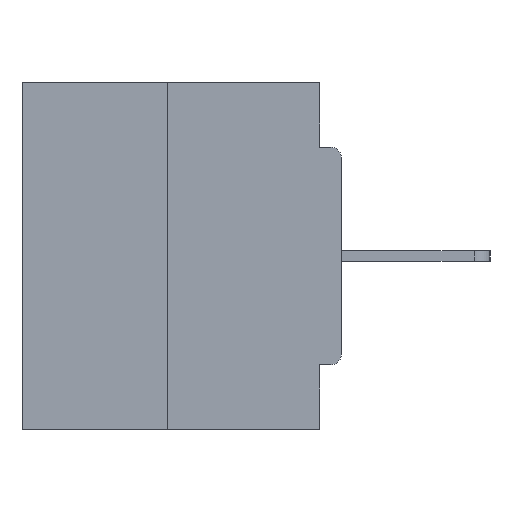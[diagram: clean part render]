
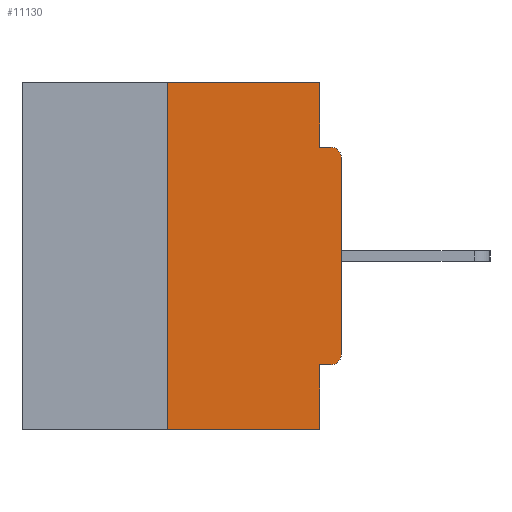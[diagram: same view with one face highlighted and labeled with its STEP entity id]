
A CAD part, left-side view. The second image highlights one B-rep face of the part: STEP entity #11130.
In plain terms, the highlighted planar face has unit normal (-1, 0, 0).
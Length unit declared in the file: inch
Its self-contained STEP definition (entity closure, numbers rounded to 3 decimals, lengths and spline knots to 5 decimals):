
#253 = CARTESIAN_POINT ( 'NONE',  ( 0., 0., 0. ) ) ;
#277 = ORIENTED_EDGE ( 'NONE', *, *, #20752, .F. ) ;
#402 = DIRECTION ( 'NONE',  ( 0., -1., 0. ) ) ;
#675 = DIRECTION ( 'NONE',  ( 0., 0., 1. ) ) ;
#771 = LINE ( 'NONE', #26077, #10764 ) ;
#1321 = VECTOR ( 'NONE', #22641, 39.37008 ) ;
#2337 = VERTEX_POINT ( 'NONE', #20572 ) ;
#3588 = CIRCLE ( 'NONE', #19612, 0.015 ) ;
#3824 = FACE_OUTER_BOUND ( 'NONE', #23256, .T. ) ;
#4654 = LINE ( 'NONE', #253, #6382 ) ;
#5637 = DIRECTION ( 'NONE',  ( 0., -1., 0. ) ) ;
#6382 = VECTOR ( 'NONE', #675, 39.37008 ) ;
#6690 = LINE ( 'NONE', #28647, #6852 ) ;
#6852 = VECTOR ( 'NONE', #22323, 39.37008 ) ;
#6928 = VERTEX_POINT ( 'NONE', #12675 ) ;
#7060 = VERTEX_POINT ( 'NONE', #24286 ) ;
#7153 = VERTEX_POINT ( 'NONE', #20764 ) ;
#8104 = ORIENTED_EDGE ( 'NONE', *, *, #13348, .F. ) ;
#8130 = DIRECTION ( 'NONE',  ( 0., 1., 0. ) ) ;
#8298 = VERTEX_POINT ( 'NONE', #16218 ) ;
#8921 = VECTOR ( 'NONE', #8130, 39.37008 ) ;
#9485 = EDGE_CURVE ( 'NONE', #28665, #2337, #20408, .T. ) ;
#10111 = DIRECTION ( 'NONE',  ( 0., 0., -1. ) ) ;
#10588 = DIRECTION ( 'NONE',  ( 0., 0., -1. ) ) ;
#10665 = CARTESIAN_POINT ( 'NONE',  ( 0., 0.015, -0.1085 ) ) ;
#10764 = VECTOR ( 'NONE', #23719, 39.37008 ) ;
#10815 = DIRECTION ( 'NONE',  ( -1., 0., 0. ) ) ;
#11130 = ADVANCED_FACE ( 'NONE', ( #3824 ), #12814, .F. ) ;
#11591 = LINE ( 'NONE', #20735, #1321 ) ;
#11714 = EDGE_CURVE ( 'NONE', #2337, #20192, #4654, .T. ) ;
#12382 = CARTESIAN_POINT ( 'NONE',  ( 0., 0.031, -0.4065 ) ) ;
#12442 = CARTESIAN_POINT ( 'NONE',  ( 0., 0.25, 0. ) ) ;
#12469 = CARTESIAN_POINT ( 'NONE',  ( 0., 0.031, -0.5 ) ) ;
#12675 = CARTESIAN_POINT ( 'NONE',  ( 0., 0.015, -0.0935 ) ) ;
#12814 = PLANE ( 'NONE',  #23311 ) ;
#12928 = ORIENTED_EDGE ( 'NONE', *, *, #11714, .T. ) ;
#13061 = EDGE_CURVE ( 'NONE', #8298, #7153, #21163, .T. ) ;
#13192 = DIRECTION ( 'NONE',  ( 0., 0., -1. ) ) ;
#13348 = EDGE_CURVE ( 'NONE', #20266, #7060, #6690, .T. ) ;
#13528 = ORIENTED_EDGE ( 'NONE', *, *, #24818, .F. ) ;
#14208 = ORIENTED_EDGE ( 'NONE', *, *, #13061, .T. ) ;
#14288 = AXIS2_PLACEMENT_3D ( 'NONE', #15085, #24336, #15395 ) ;
#14885 = CARTESIAN_POINT ( 'NONE',  ( 0., 0.46, 0. ) ) ;
#15014 = ORIENTED_EDGE ( 'NONE', *, *, #9485, .T. ) ;
#15085 = CARTESIAN_POINT ( 'NONE',  ( 0., 0.015, -0.3915 ) ) ;
#15395 = DIRECTION ( 'NONE',  ( 0., 0., -1. ) ) ;
#16218 = CARTESIAN_POINT ( 'NONE',  ( 0., 0.25, -0.5 ) ) ;
#16413 = CARTESIAN_POINT ( 'NONE',  ( 0., 0., -0.0935 ) ) ;
#18247 = CARTESIAN_POINT ( 'NONE',  ( 0., 0.46, -0.5 ) ) ;
#18319 = ORIENTED_EDGE ( 'NONE', *, *, #21670, .T. ) ;
#18381 = ORIENTED_EDGE ( 'NONE', *, *, #23871, .F. ) ;
#18472 = LINE ( 'NONE', #16413, #22472 ) ;
#19612 = AXIS2_PLACEMENT_3D ( 'NONE', #10665, #10815, #13192 ) ;
#19864 = CARTESIAN_POINT ( 'NONE',  ( 0., 0.015, -0.4065 ) ) ;
#20192 = VERTEX_POINT ( 'NONE', #20571 ) ;
#20266 = VERTEX_POINT ( 'NONE', #12442 ) ;
#20408 = CIRCLE ( 'NONE', #14288, 0.015 ) ;
#20571 = CARTESIAN_POINT ( 'NONE',  ( 0., 0., -0.1085 ) ) ;
#20572 = CARTESIAN_POINT ( 'NONE',  ( 0., 0., -0.3915 ) ) ;
#20735 = CARTESIAN_POINT ( 'NONE',  ( 0., 0.25, 0. ) ) ;
#20752 = EDGE_CURVE ( 'NONE', #24658, #6928, #18472, .T. ) ;
#20764 = CARTESIAN_POINT ( 'NONE',  ( 0., 0.031, -0.5 ) ) ;
#21148 = ORIENTED_EDGE ( 'NONE', *, *, #28751, .F. ) ;
#21163 = LINE ( 'NONE', #18247, #28953 ) ;
#21670 = EDGE_CURVE ( 'NONE', #20192, #6928, #3588, .T. ) ;
#22323 = DIRECTION ( 'NONE',  ( 0., -1., 0. ) ) ;
#22472 = VECTOR ( 'NONE', #5637, 39.37008 ) ;
#22641 = DIRECTION ( 'NONE',  ( 0., 0., 1. ) ) ;
#23256 = EDGE_LOOP ( 'NONE', ( #8104, #21148, #14208, #25121, #13528, #15014, #12928, #18319, #277, #18381 ) ) ;
#23311 = AXIS2_PLACEMENT_3D ( 'NONE', #14885, #25775, #10588 ) ;
#23511 = LINE ( 'NONE', #12469, #25900 ) ;
#23719 = DIRECTION ( 'NONE',  ( 0., 0., -1. ) ) ;
#23871 = EDGE_CURVE ( 'NONE', #7060, #24658, #771, .T. ) ;
#24286 = CARTESIAN_POINT ( 'NONE',  ( 0., 0.031, 0. ) ) ;
#24336 = DIRECTION ( 'NONE',  ( -1., 0., 0. ) ) ;
#24658 = VERTEX_POINT ( 'NONE', #25097 ) ;
#24818 = EDGE_CURVE ( 'NONE', #28665, #26866, #25977, .T. ) ;
#25097 = CARTESIAN_POINT ( 'NONE',  ( 0., 0.031, -0.0935 ) ) ;
#25121 = ORIENTED_EDGE ( 'NONE', *, *, #25656, .F. ) ;
#25656 = EDGE_CURVE ( 'NONE', #26866, #7153, #23511, .T. ) ;
#25775 = DIRECTION ( 'NONE',  ( 1., 0., 0. ) ) ;
#25900 = VECTOR ( 'NONE', #10111, 39.37008 ) ;
#25977 = LINE ( 'NONE', #27893, #8921 ) ;
#26077 = CARTESIAN_POINT ( 'NONE',  ( 0., 0.031, 0. ) ) ;
#26866 = VERTEX_POINT ( 'NONE', #12382 ) ;
#27893 = CARTESIAN_POINT ( 'NONE',  ( 0., 0., -0.4065 ) ) ;
#28647 = CARTESIAN_POINT ( 'NONE',  ( 0., 0.46, 0. ) ) ;
#28665 = VERTEX_POINT ( 'NONE', #19864 ) ;
#28751 = EDGE_CURVE ( 'NONE', #8298, #20266, #11591, .T. ) ;
#28953 = VECTOR ( 'NONE', #402, 39.37008 ) ;
